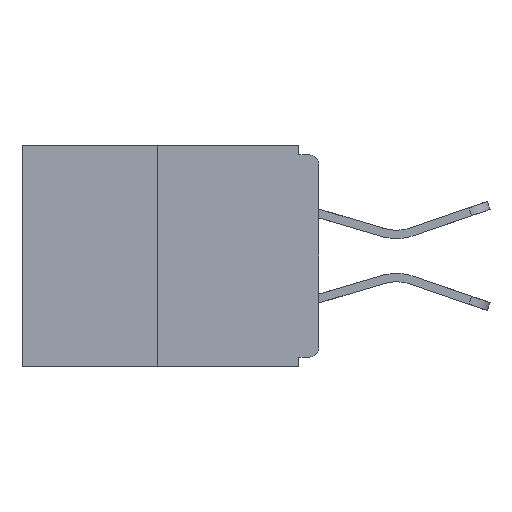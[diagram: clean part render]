
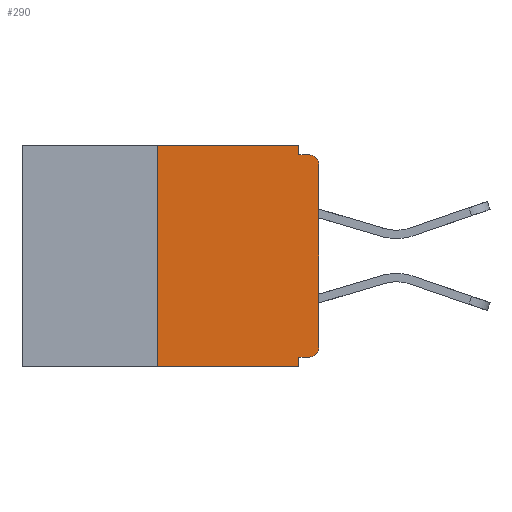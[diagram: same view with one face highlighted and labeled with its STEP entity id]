
A CAD part, left-side view. The second image highlights one B-rep face of the part: STEP entity #290.
In plain terms, the highlighted planar face has unit normal (-1, 0, 0).
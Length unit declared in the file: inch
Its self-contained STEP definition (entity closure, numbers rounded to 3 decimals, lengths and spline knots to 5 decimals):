
#290 = ADVANCED_FACE ( 'NONE', ( #14915 ), #9197, .F. ) ;
#382 = CIRCLE ( 'NONE', #22997, 0.015 ) ;
#690 = LINE ( 'NONE', #10436, #18760 ) ;
#847 = CARTESIAN_POINT ( 'NONE',  ( 0., 0.031, -0.015 ) ) ;
#861 = EDGE_CURVE ( 'NONE', #27649, #5054, #26428, .T. ) ;
#1116 = ORIENTED_EDGE ( 'NONE', *, *, #3862, .T. ) ;
#1121 = EDGE_CURVE ( 'NONE', #13102, #24693, #17690, .T. ) ;
#1377 = VECTOR ( 'NONE', #11576, 39.37008 ) ;
#1504 = DIRECTION ( 'NONE',  ( 0., 0., -1. ) ) ;
#1583 = CARTESIAN_POINT ( 'NONE',  ( 0., 0.015, -0.313 ) ) ;
#1648 = VERTEX_POINT ( 'NONE', #13459 ) ;
#2248 = EDGE_CURVE ( 'NONE', #12427, #27649, #9236, .T. ) ;
#2297 = VECTOR ( 'NONE', #3291, 39.37008 ) ;
#2730 = CIRCLE ( 'NONE', #10595, 0.015 ) ;
#2763 = VERTEX_POINT ( 'NONE', #6168 ) ;
#3291 = DIRECTION ( 'NONE',  ( 0., 0., 1. ) ) ;
#3862 = EDGE_CURVE ( 'NONE', #1648, #8251, #382, .T. ) ;
#3901 = ORIENTED_EDGE ( 'NONE', *, *, #25546, .F. ) ;
#3921 = DIRECTION ( 'NONE',  ( -1., 0., 0. ) ) ;
#4524 = DIRECTION ( 'NONE',  ( 1., 0., 0. ) ) ;
#4769 = EDGE_LOOP ( 'NONE', ( #18369, #5338, #20180, #3901, #27789, #1116, #10451, #17795, #24168, #14340 ) ) ;
#4835 = CARTESIAN_POINT ( 'NONE',  ( 0., 0.031, 0. ) ) ;
#5054 = VERTEX_POINT ( 'NONE', #4835 ) ;
#5153 = VECTOR ( 'NONE', #15242, 39.37008 ) ;
#5338 = ORIENTED_EDGE ( 'NONE', *, *, #2248, .F. ) ;
#5405 = EDGE_CURVE ( 'NONE', #2763, #24693, #2730, .T. ) ;
#5707 = CARTESIAN_POINT ( 'NONE',  ( 0., 0.46, 0. ) ) ;
#6060 = CARTESIAN_POINT ( 'NONE',  ( 0., 0.015, -0.03 ) ) ;
#6168 = CARTESIAN_POINT ( 'NONE',  ( 0., 0., -0.03 ) ) ;
#6469 = CARTESIAN_POINT ( 'NONE',  ( 0., 0., -0.015 ) ) ;
#6563 = LINE ( 'NONE', #7069, #1377 ) ;
#6768 = VECTOR ( 'NONE', #12097, 39.37008 ) ;
#7069 = CARTESIAN_POINT ( 'NONE',  ( 0., 0.031, -0.343 ) ) ;
#7758 = EDGE_CURVE ( 'NONE', #8251, #2763, #24882, .T. ) ;
#8251 = VERTEX_POINT ( 'NONE', #25739 ) ;
#8915 = CARTESIAN_POINT ( 'NONE',  ( 0., 0., -0.328 ) ) ;
#9110 = DIRECTION ( 'NONE',  ( 0., 0., 1. ) ) ;
#9197 = PLANE ( 'NONE',  #15103 ) ;
#9236 = LINE ( 'NONE', #21093, #2297 ) ;
#10436 = CARTESIAN_POINT ( 'NONE',  ( 0., 0.46, -0.343 ) ) ;
#10451 = ORIENTED_EDGE ( 'NONE', *, *, #7758, .T. ) ;
#10595 = AXIS2_PLACEMENT_3D ( 'NONE', #6060, #3921, #1504 ) ;
#11123 = EDGE_CURVE ( 'NONE', #1648, #22771, #27604, .T. ) ;
#11178 = CARTESIAN_POINT ( 'NONE',  ( 0., 0.031, -0.328 ) ) ;
#11576 = DIRECTION ( 'NONE',  ( 0., 0., -1. ) ) ;
#12097 = DIRECTION ( 'NONE',  ( 0., 0., -1. ) ) ;
#12427 = VERTEX_POINT ( 'NONE', #22316 ) ;
#13102 = VERTEX_POINT ( 'NONE', #847 ) ;
#13459 = CARTESIAN_POINT ( 'NONE',  ( 0., 0.015, -0.328 ) ) ;
#13677 = DIRECTION ( 'NONE',  ( 0., 0., -1. ) ) ;
#14340 = ORIENTED_EDGE ( 'NONE', *, *, #22486, .F. ) ;
#14573 = DIRECTION ( 'NONE',  ( 0., -1., 0. ) ) ;
#14915 = FACE_OUTER_BOUND ( 'NONE', #4769, .T. ) ;
#15103 = AXIS2_PLACEMENT_3D ( 'NONE', #17851, #4524, #13677 ) ;
#15242 = DIRECTION ( 'NONE',  ( 0., -1., 0. ) ) ;
#15810 = VERTEX_POINT ( 'NONE', #27488 ) ;
#17146 = DIRECTION ( 'NONE',  ( -1., 0., 0. ) ) ;
#17690 = LINE ( 'NONE', #6469, #5153 ) ;
#17795 = ORIENTED_EDGE ( 'NONE', *, *, #5405, .T. ) ;
#17851 = CARTESIAN_POINT ( 'NONE',  ( 0., 0.46, 0. ) ) ;
#18369 = ORIENTED_EDGE ( 'NONE', *, *, #861, .F. ) ;
#18760 = VECTOR ( 'NONE', #19727, 39.37008 ) ;
#19357 = DIRECTION ( 'NONE',  ( 0., 0., -1. ) ) ;
#19727 = DIRECTION ( 'NONE',  ( 0., -1., 0. ) ) ;
#20180 = ORIENTED_EDGE ( 'NONE', *, *, #25287, .T. ) ;
#20727 = CARTESIAN_POINT ( 'NONE',  ( 0., 0.015, -0.015 ) ) ;
#21093 = CARTESIAN_POINT ( 'NONE',  ( 0., 0.25, 0. ) ) ;
#22316 = CARTESIAN_POINT ( 'NONE',  ( 0., 0.25, -0.343 ) ) ;
#22349 = DIRECTION ( 'NONE',  ( 0., 1., 0. ) ) ;
#22486 = EDGE_CURVE ( 'NONE', #5054, #13102, #26294, .T. ) ;
#22771 = VERTEX_POINT ( 'NONE', #11178 ) ;
#22997 = AXIS2_PLACEMENT_3D ( 'NONE', #1583, #17146, #19357 ) ;
#24168 = ORIENTED_EDGE ( 'NONE', *, *, #1121, .F. ) ;
#24502 = CARTESIAN_POINT ( 'NONE',  ( 0., 0., 0. ) ) ;
#24693 = VERTEX_POINT ( 'NONE', #20727 ) ;
#24882 = LINE ( 'NONE', #24502, #26607 ) ;
#25287 = EDGE_CURVE ( 'NONE', #12427, #15810, #690, .T. ) ;
#25546 = EDGE_CURVE ( 'NONE', #22771, #15810, #6563, .T. ) ;
#25716 = VECTOR ( 'NONE', #14573, 39.37008 ) ;
#25739 = CARTESIAN_POINT ( 'NONE',  ( 0., 0., -0.313 ) ) ;
#26294 = LINE ( 'NONE', #27545, #6768 ) ;
#26428 = LINE ( 'NONE', #5707, #25716 ) ;
#26607 = VECTOR ( 'NONE', #9110, 39.37008 ) ;
#27134 = CARTESIAN_POINT ( 'NONE',  ( 0., 0.25, 0. ) ) ;
#27488 = CARTESIAN_POINT ( 'NONE',  ( 0., 0.031, -0.343 ) ) ;
#27545 = CARTESIAN_POINT ( 'NONE',  ( 0., 0.031, 0. ) ) ;
#27604 = LINE ( 'NONE', #8915, #28323 ) ;
#27649 = VERTEX_POINT ( 'NONE', #27134 ) ;
#27789 = ORIENTED_EDGE ( 'NONE', *, *, #11123, .F. ) ;
#28323 = VECTOR ( 'NONE', #22349, 39.37008 ) ;
